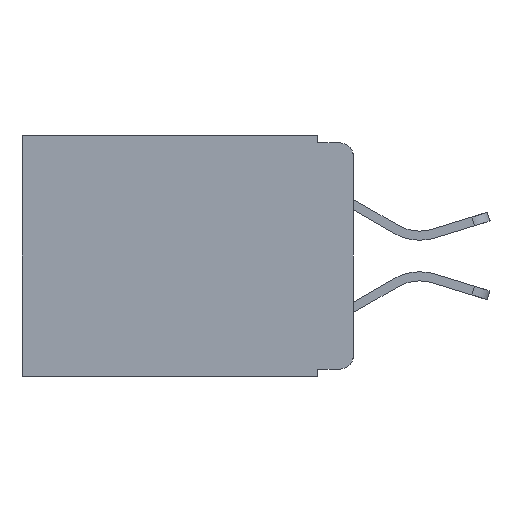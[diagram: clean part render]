
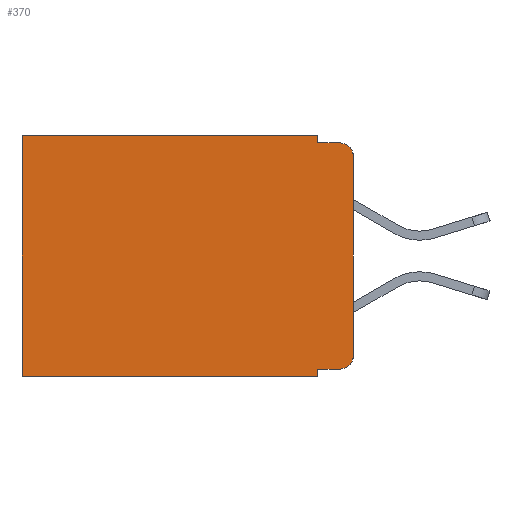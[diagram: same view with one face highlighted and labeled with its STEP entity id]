
A CAD part, left-side view. The second image highlights one B-rep face of the part: STEP entity #370.
In plain terms, the highlighted planar face has unit normal (-1, 0, 0).
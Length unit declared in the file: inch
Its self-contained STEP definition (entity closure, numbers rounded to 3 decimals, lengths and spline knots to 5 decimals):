
#59 = ORIENTED_EDGE ( 'NONE', *, *, #9792, .F. ) ;
#108 = CARTESIAN_POINT ( 'NONE',  ( 0.298, 0., 0. ) ) ;
#236 = ORIENTED_EDGE ( 'NONE', *, *, #9317, .T. ) ;
#357 = VERTEX_POINT ( 'NONE', #647 ) ;
#370 = ADVANCED_FACE ( 'NONE', ( #4522 ), #6181, .F. ) ;
#440 = VERTEX_POINT ( 'NONE', #3952 ) ;
#647 = CARTESIAN_POINT ( 'NONE',  ( 0.298, 0.02, -0.01 ) ) ;
#666 = DIRECTION ( 'NONE',  ( 0., 0., -1. ) ) ;
#965 = EDGE_CURVE ( 'NONE', #7581, #4605, #5693, .T. ) ;
#1001 = VERTEX_POINT ( 'NONE', #1434 ) ;
#1255 = ORIENTED_EDGE ( 'NONE', *, *, #9045, .T. ) ;
#1433 = VERTEX_POINT ( 'NONE', #3783 ) ;
#1434 = CARTESIAN_POINT ( 'NONE',  ( 0.298, 0., -0.313 ) ) ;
#1700 = DIRECTION ( 'NONE',  ( 1., 0., 0. ) ) ;
#1802 = VECTOR ( 'NONE', #7746, 39.37008 ) ;
#1914 = ORIENTED_EDGE ( 'NONE', *, *, #3122, .F. ) ;
#2022 = CARTESIAN_POINT ( 'NONE',  ( 0.298, 0.051, -0.333 ) ) ;
#2044 = DIRECTION ( 'NONE',  ( 0., 0., -1. ) ) ;
#2047 = ORIENTED_EDGE ( 'NONE', *, *, #8599, .T. ) ;
#2127 = CARTESIAN_POINT ( 'NONE',  ( 0.298, 0.02, -0.333 ) ) ;
#2182 = CARTESIAN_POINT ( 'NONE',  ( 0.298, 0.051, -0.01 ) ) ;
#2240 = VECTOR ( 'NONE', #2044, 39.37008 ) ;
#2275 = DIRECTION ( 'NONE',  ( 0., -1., 0. ) ) ;
#2307 = DIRECTION ( 'NONE',  ( -1., 0., 0. ) ) ;
#2376 = LINE ( 'NONE', #7671, #9938 ) ;
#3046 = DIRECTION ( 'NONE',  ( 0., 0., -1. ) ) ;
#3122 = EDGE_CURVE ( 'NONE', #5923, #9175, #4021, .T. ) ;
#3124 = VECTOR ( 'NONE', #9628, 39.37008 ) ;
#3363 = ORIENTED_EDGE ( 'NONE', *, *, #5072, .F. ) ;
#3466 = LINE ( 'NONE', #2182, #5551 ) ;
#3479 = EDGE_LOOP ( 'NONE', ( #5353, #3684, #3363, #4229, #3686, #236, #59, #1914, #1255, #2047 ) ) ;
#3626 = VECTOR ( 'NONE', #7922, 39.37008 ) ;
#3632 = AXIS2_PLACEMENT_3D ( 'NONE', #9835, #5680, #666 ) ;
#3684 = ORIENTED_EDGE ( 'NONE', *, *, #6742, .T. ) ;
#3686 = ORIENTED_EDGE ( 'NONE', *, *, #965, .T. ) ;
#3770 = AXIS2_PLACEMENT_3D ( 'NONE', #4063, #1700, #6981 ) ;
#3783 = CARTESIAN_POINT ( 'NONE',  ( 0.298, 0., -0.03 ) ) ;
#3952 = CARTESIAN_POINT ( 'NONE',  ( 0.298, 0.051, -0.01 ) ) ;
#4021 = LINE ( 'NONE', #9961, #3124 ) ;
#4063 = CARTESIAN_POINT ( 'NONE',  ( 0.298, 0., 0. ) ) ;
#4142 = VECTOR ( 'NONE', #8609, 39.37008 ) ;
#4229 = ORIENTED_EDGE ( 'NONE', *, *, #6093, .F. ) ;
#4326 = LINE ( 'NONE', #8946, #8222 ) ;
#4522 = FACE_OUTER_BOUND ( 'NONE', #3479, .T. ) ;
#4605 = VERTEX_POINT ( 'NONE', #5388 ) ;
#5072 = EDGE_CURVE ( 'NONE', #440, #357, #3466, .T. ) ;
#5353 = ORIENTED_EDGE ( 'NONE', *, *, #9596, .F. ) ;
#5388 = CARTESIAN_POINT ( 'NONE',  ( 0.298, 0.473, 0. ) ) ;
#5551 = VECTOR ( 'NONE', #9928, 39.37008 ) ;
#5680 = DIRECTION ( 'NONE',  ( -1., 0., 0. ) ) ;
#5693 = LINE ( 'NONE', #108, #3626 ) ;
#5763 = CARTESIAN_POINT ( 'NONE',  ( 0.298, 0., -0.343 ) ) ;
#5923 = VERTEX_POINT ( 'NONE', #2022 ) ;
#6093 = EDGE_CURVE ( 'NONE', #7581, #440, #4326, .T. ) ;
#6181 = PLANE ( 'NONE',  #3770 ) ;
#6192 = LINE ( 'NONE', #5763, #4142 ) ;
#6451 = LINE ( 'NONE', #6778, #2240 ) ;
#6626 = VERTEX_POINT ( 'NONE', #2127 ) ;
#6742 = EDGE_CURVE ( 'NONE', #1433, #357, #9786, .T. ) ;
#6778 = CARTESIAN_POINT ( 'NONE',  ( 0.298, 0.473, 0. ) ) ;
#6981 = DIRECTION ( 'NONE',  ( 0., 0., -1. ) ) ;
#6986 = CARTESIAN_POINT ( 'NONE',  ( 0.298, 0.02, -0.03 ) ) ;
#7040 = CARTESIAN_POINT ( 'NONE',  ( 0.298, 0., 0. ) ) ;
#7581 = VERTEX_POINT ( 'NONE', #9014 ) ;
#7671 = CARTESIAN_POINT ( 'NONE',  ( 0.298, 0.051, -0.333 ) ) ;
#7698 = DIRECTION ( 'NONE',  ( 0., 0., -1. ) ) ;
#7746 = DIRECTION ( 'NONE',  ( 0., 0., -1. ) ) ;
#7922 = DIRECTION ( 'NONE',  ( 0., 1., 0. ) ) ;
#8171 = LINE ( 'NONE', #7040, #1802 ) ;
#8222 = VECTOR ( 'NONE', #3046, 39.37008 ) ;
#8404 = CIRCLE ( 'NONE', #3632, 0.02 ) ;
#8599 = EDGE_CURVE ( 'NONE', #6626, #1001, #8404, .T. ) ;
#8609 = DIRECTION ( 'NONE',  ( 0., 1., 0. ) ) ;
#8946 = CARTESIAN_POINT ( 'NONE',  ( 0.298, 0.051, 0. ) ) ;
#9014 = CARTESIAN_POINT ( 'NONE',  ( 0.298, 0.051, 0. ) ) ;
#9045 = EDGE_CURVE ( 'NONE', #5923, #6626, #2376, .T. ) ;
#9175 = VERTEX_POINT ( 'NONE', #9364 ) ;
#9317 = EDGE_CURVE ( 'NONE', #4605, #9996, #6451, .T. ) ;
#9364 = CARTESIAN_POINT ( 'NONE',  ( 0.298, 0.051, -0.343 ) ) ;
#9494 = CARTESIAN_POINT ( 'NONE',  ( 0.298, 0.473, -0.343 ) ) ;
#9499 = AXIS2_PLACEMENT_3D ( 'NONE', #6986, #2307, #7698 ) ;
#9596 = EDGE_CURVE ( 'NONE', #1433, #1001, #8171, .T. ) ;
#9628 = DIRECTION ( 'NONE',  ( 0., 0., -1. ) ) ;
#9786 = CIRCLE ( 'NONE', #9499, 0.02 ) ;
#9792 = EDGE_CURVE ( 'NONE', #9175, #9996, #6192, .T. ) ;
#9835 = CARTESIAN_POINT ( 'NONE',  ( 0.298, 0.02, -0.313 ) ) ;
#9928 = DIRECTION ( 'NONE',  ( 0., -1., 0. ) ) ;
#9938 = VECTOR ( 'NONE', #2275, 39.37008 ) ;
#9961 = CARTESIAN_POINT ( 'NONE',  ( 0.298, 0.051, 0. ) ) ;
#9996 = VERTEX_POINT ( 'NONE', #9494 ) ;
